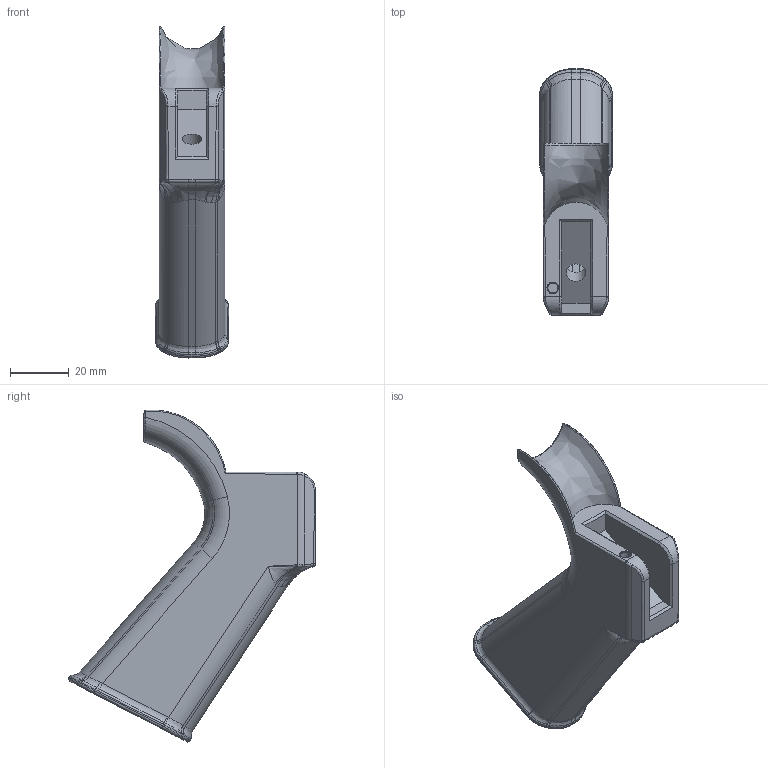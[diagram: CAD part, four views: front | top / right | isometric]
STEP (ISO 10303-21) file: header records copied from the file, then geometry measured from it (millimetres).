
FILE_DESCRIPTION(/* description */ (''),/* implementation_level */ '2;1');
FILE_NAME(/* name */ 'Standard.step',/* time_stamp */ '2021-09-05T14:41:04-04:00',/* author */ (''),/* organization */ (''),/* preprocessor_version */ 'ST-DEVELOPER v18.1',/* originating_system */ 'Autodesk Translation Framework v10.10.0.1391',/* authorisation */ '');
FILE_SCHEMA (('AUTOMOTIVE_DESIGN { 1 0 10303 214 3 1 1 }'));
Length unit declared in the file: millimetre
Products named in the file (1): Standard
Bounding box: 24.83 x 83.89 x 112.88 mm (x, y, z)
Volume: 47869.1 mm3; surface area: 20653.1 mm2
Topology: 1 solids, 1 shells, 308 faces, 717 edges, 408 vertices
Faces by surface type: bspline 164, cylinder 63, plane 56, torus 17, cone 8
Full cylindrical faces by diameter (mm): 3.4 x1, 6.8 x1, 14.521 x1, 16.771 x1
Entity records: 13728 total; most frequent: CARTESIAN_POINT 7734, ORIENTED_EDGE 1414, DIRECTION 913, EDGE_CURVE 707, VERTEX_POINT 408, AXIS2_PLACEMENT_3D 359, EDGE_LOOP 317, FACE_OUTER_BOUND 308
